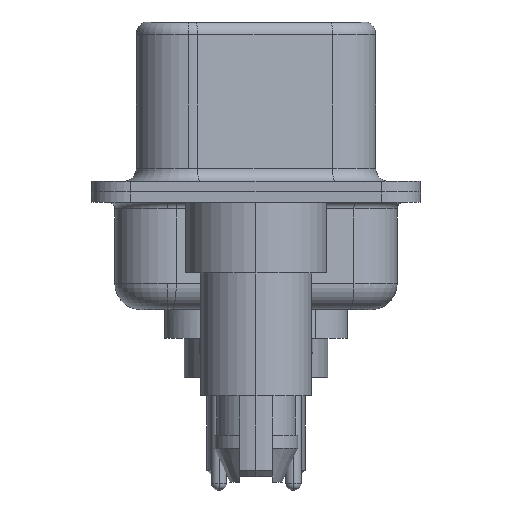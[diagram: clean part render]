
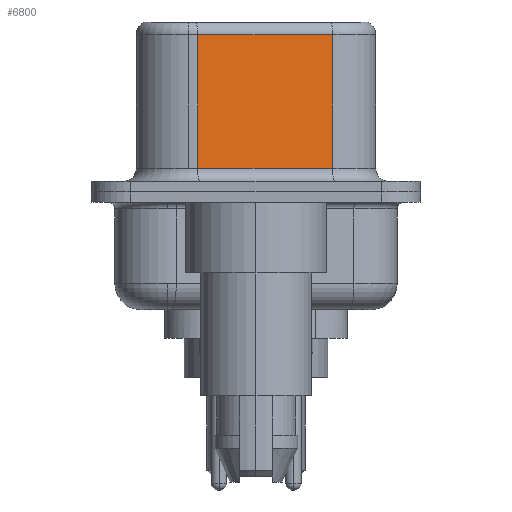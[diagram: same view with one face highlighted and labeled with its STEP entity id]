
A CAD part, left-side view. The second image highlights one B-rep face of the part: STEP entity #6800.
In plain terms, the highlighted planar face has unit normal (-0.985, -0.174, 0).
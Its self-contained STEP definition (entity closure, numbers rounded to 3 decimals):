
#244 = DIRECTION ( 'NONE',  ( 0.174, -0.985, 0. ) ) ;
#258 = CARTESIAN_POINT ( 'NONE',  ( 3.67, 2.233, 6.52 ) ) ;
#418 = CARTESIAN_POINT ( 'NONE',  ( 4.58, -2.927, 6.02 ) ) ;
#942 = ORIENTED_EDGE ( 'NONE', *, *, #13663, .F. ) ;
#1232 = CARTESIAN_POINT ( 'NONE',  ( 3.67, 2.233, 0.9 ) ) ;
#1487 = VECTOR ( 'NONE', #14290, 1000. ) ;
#1553 = FACE_OUTER_BOUND ( 'NONE', #3538, .T. ) ;
#2343 = PLANE ( 'NONE',  #11335 ) ;
#2463 = VERTEX_POINT ( 'NONE', #14491 ) ;
#3518 = DIRECTION ( 'NONE',  ( 0.985, 0.174, 0. ) ) ;
#3538 = EDGE_LOOP ( 'NONE', ( #942, #11259, #13348, #10622 ) ) ;
#3898 = CARTESIAN_POINT ( 'NONE',  ( 4.58, -2.927, 6.52 ) ) ;
#4036 = CARTESIAN_POINT ( 'NONE',  ( 4.58, -2.927, 6.02 ) ) ;
#4241 = VERTEX_POINT ( 'NONE', #4036 ) ;
#4609 = LINE ( 'NONE', #258, #7280 ) ;
#4640 = EDGE_CURVE ( 'NONE', #14025, #6983, #6064, .T. ) ;
#6064 = LINE ( 'NONE', #9437, #12200 ) ;
#6150 = EDGE_CURVE ( 'NONE', #2463, #14025, #4609, .T. ) ;
#6298 = EDGE_CURVE ( 'NONE', #4241, #2463, #12357, .T. ) ;
#6800 = ADVANCED_FACE ( 'NONE', ( #1553 ), #2343, .F. ) ;
#6983 = VERTEX_POINT ( 'NONE', #8590 ) ;
#7280 = VECTOR ( 'NONE', #8308, 1000. ) ;
#8308 = DIRECTION ( 'NONE',  ( 0., 0., -1. ) ) ;
#8590 = CARTESIAN_POINT ( 'NONE',  ( 4.58, -2.927, 0.9 ) ) ;
#9437 = CARTESIAN_POINT ( 'NONE',  ( 4.58, -2.927, 0.9 ) ) ;
#10622 = ORIENTED_EDGE ( 'NONE', *, *, #4640, .T. ) ;
#10730 = DIRECTION ( 'NONE',  ( -0.174, 0.985, 0. ) ) ;
#11259 = ORIENTED_EDGE ( 'NONE', *, *, #6298, .T. ) ;
#11335 = AXIS2_PLACEMENT_3D ( 'NONE', #13714, #3518, #11547 ) ;
#11547 = DIRECTION ( 'NONE',  ( -0.174, 0.985, 0. ) ) ;
#11979 = VECTOR ( 'NONE', #10730, 1000. ) ;
#12200 = VECTOR ( 'NONE', #244, 1000. ) ;
#12357 = LINE ( 'NONE', #418, #11979 ) ;
#13348 = ORIENTED_EDGE ( 'NONE', *, *, #6150, .T. ) ;
#13663 = EDGE_CURVE ( 'NONE', #4241, #6983, #13718, .T. ) ;
#13714 = CARTESIAN_POINT ( 'NONE',  ( 4.58, -2.927, 6.52 ) ) ;
#13718 = LINE ( 'NONE', #3898, #1487 ) ;
#14025 = VERTEX_POINT ( 'NONE', #1232 ) ;
#14290 = DIRECTION ( 'NONE',  ( 0., 0., -1. ) ) ;
#14491 = CARTESIAN_POINT ( 'NONE',  ( 3.67, 2.233, 6.02 ) ) ;
